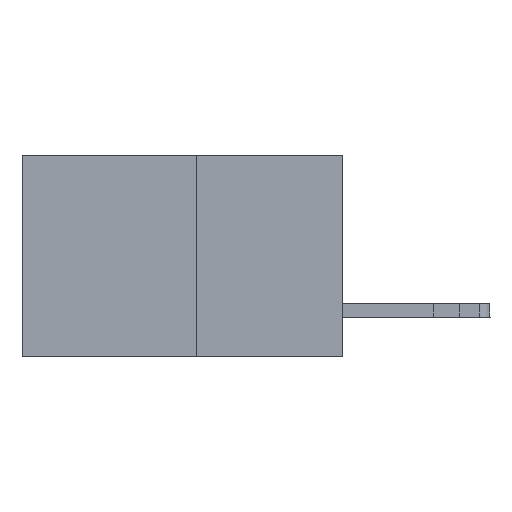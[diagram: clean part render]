
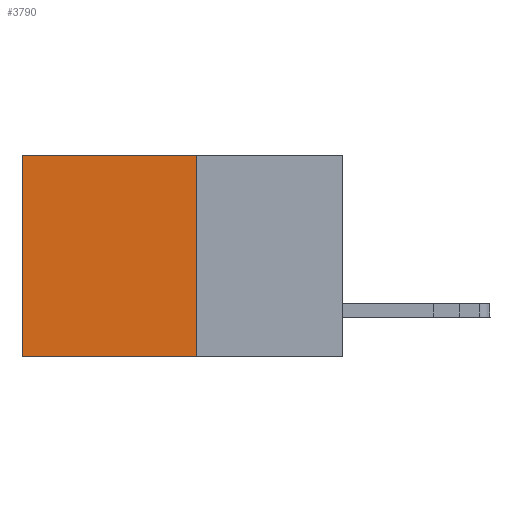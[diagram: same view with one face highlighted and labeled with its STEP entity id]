
A CAD part, left-side view. The second image highlights one B-rep face of the part: STEP entity #3790.
In plain terms, the highlighted planar face has unit normal (-1, 0, 0).
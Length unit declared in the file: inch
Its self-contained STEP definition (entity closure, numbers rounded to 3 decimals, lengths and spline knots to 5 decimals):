
#74 = CARTESIAN_POINT ( 'NONE',  ( 0.277, 0.27, -0.37 ) ) ;
#568 = VERTEX_POINT ( 'NONE', #1203 ) ;
#1152 = DIRECTION ( 'NONE',  ( 0., 0., -1. ) ) ;
#1191 = EDGE_CURVE ( 'NONE', #12607, #7876, #4833, .T. ) ;
#1203 = CARTESIAN_POINT ( 'NONE',  ( 0.277, 0.27, 0. ) ) ;
#1435 = CARTESIAN_POINT ( 'NONE',  ( 0.277, 0.27, -0.37 ) ) ;
#1482 = VERTEX_POINT ( 'NONE', #9519 ) ;
#2199 = AXIS2_PLACEMENT_3D ( 'NONE', #4590, #12232, #1152 ) ;
#2458 = ORIENTED_EDGE ( 'NONE', *, *, #4427, .T. ) ;
#2707 = DIRECTION ( 'NONE',  ( 0., 1., 0. ) ) ;
#2743 = LINE ( 'NONE', #6114, #5932 ) ;
#3169 = VECTOR ( 'NONE', #2707, 39.37008 ) ;
#3780 = ORIENTED_EDGE ( 'NONE', *, *, #8375, .T. ) ;
#3790 = ADVANCED_FACE ( 'NONE', ( #7898 ), #12097, .F. ) ;
#4245 = LINE ( 'NONE', #74, #12350 ) ;
#4427 = EDGE_CURVE ( 'NONE', #1482, #7876, #9642, .T. ) ;
#4590 = CARTESIAN_POINT ( 'NONE',  ( 0.277, 0.27, -0.37 ) ) ;
#4833 = LINE ( 'NONE', #12149, #3169 ) ;
#5411 = DIRECTION ( 'NONE',  ( 0., 0., -1. ) ) ;
#5932 = VECTOR ( 'NONE', #9008, 39.37008 ) ;
#6114 = CARTESIAN_POINT ( 'NONE',  ( 0.277, 0.27, 0. ) ) ;
#6823 = CARTESIAN_POINT ( 'NONE',  ( 0.277, 0.59, -0.37 ) ) ;
#7876 = VERTEX_POINT ( 'NONE', #6823 ) ;
#7898 = FACE_OUTER_BOUND ( 'NONE', #13169, .T. ) ;
#8375 = EDGE_CURVE ( 'NONE', #568, #1482, #2743, .T. ) ;
#9008 = DIRECTION ( 'NONE',  ( 0., 1., 0. ) ) ;
#9519 = CARTESIAN_POINT ( 'NONE',  ( 0.277, 0.59, 0. ) ) ;
#9642 = LINE ( 'NONE', #12825, #11698 ) ;
#11505 = ORIENTED_EDGE ( 'NONE', *, *, #12083, .F. ) ;
#11698 = VECTOR ( 'NONE', #11928, 39.37008 ) ;
#11928 = DIRECTION ( 'NONE',  ( 0., 0., -1. ) ) ;
#12083 = EDGE_CURVE ( 'NONE', #568, #12607, #4245, .T. ) ;
#12097 = PLANE ( 'NONE',  #2199 ) ;
#12149 = CARTESIAN_POINT ( 'NONE',  ( 0.277, 0.27, -0.37 ) ) ;
#12210 = ORIENTED_EDGE ( 'NONE', *, *, #1191, .F. ) ;
#12232 = DIRECTION ( 'NONE',  ( 1., 0., 0. ) ) ;
#12350 = VECTOR ( 'NONE', #5411, 39.37008 ) ;
#12607 = VERTEX_POINT ( 'NONE', #1435 ) ;
#12825 = CARTESIAN_POINT ( 'NONE',  ( 0.277, 0.59, -0.37 ) ) ;
#13169 = EDGE_LOOP ( 'NONE', ( #2458, #12210, #11505, #3780 ) ) ;
